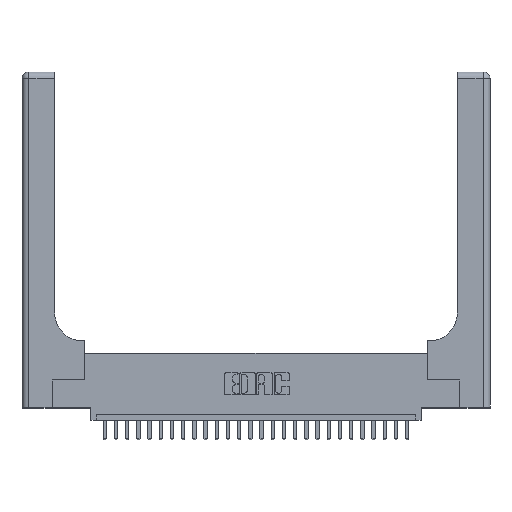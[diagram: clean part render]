
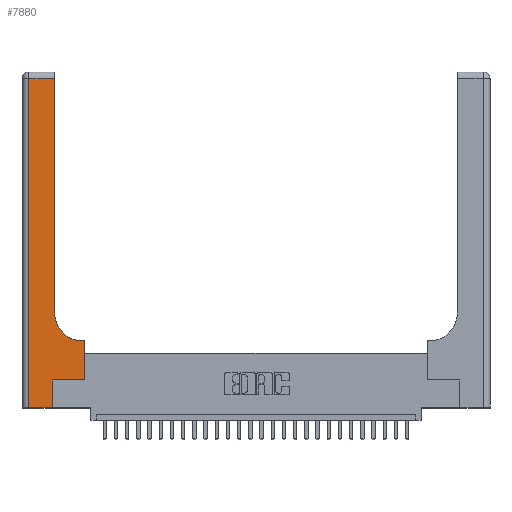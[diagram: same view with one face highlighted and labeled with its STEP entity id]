
A CAD part, top view. The second image highlights one B-rep face of the part: STEP entity #7880.
In plain terms, the highlighted planar face has unit normal (0, 0, 1).
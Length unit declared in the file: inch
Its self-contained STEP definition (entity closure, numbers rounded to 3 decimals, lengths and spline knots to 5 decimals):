
#289 = VECTOR ( 'NONE', #9527, 39.37008 ) ;
#341 = EDGE_CURVE ( 'NONE', #27066, #13692, #6060, .T. ) ;
#349 = ORIENTED_EDGE ( 'NONE', *, *, #12071, .T. ) ;
#788 = PLANE ( 'NONE',  #20138 ) ;
#1796 = VECTOR ( 'NONE', #8685, 39.37008 ) ;
#2355 = VERTEX_POINT ( 'NONE', #24753 ) ;
#2780 = VERTEX_POINT ( 'NONE', #15666 ) ;
#2901 = DIRECTION ( 'NONE',  ( 0., 0., -1. ) ) ;
#3776 = CARTESIAN_POINT ( 'NONE',  ( 0.06, 2.94, 0.37 ) ) ;
#3801 = CARTESIAN_POINT ( 'NONE',  ( 0., 0., 0.37 ) ) ;
#4126 = CARTESIAN_POINT ( 'NONE',  ( 0.06, 0., 0.37 ) ) ;
#4348 = VECTOR ( 'NONE', #10795, 39.37008 ) ;
#4604 = VERTEX_POINT ( 'NONE', #4126 ) ;
#4637 = VERTEX_POINT ( 'NONE', #7533 ) ;
#4756 = ORIENTED_EDGE ( 'NONE', *, *, #5649, .T. ) ;
#5040 = LINE ( 'NONE', #14088, #17760 ) ;
#5413 = FACE_OUTER_BOUND ( 'NONE', #22908, .T. ) ;
#5649 = EDGE_CURVE ( 'NONE', #4604, #4637, #25862, .T. ) ;
#5733 = LINE ( 'NONE', #9620, #289 ) ;
#6060 = LINE ( 'NONE', #28026, #4348 ) ;
#6322 = EDGE_CURVE ( 'NONE', #13692, #2355, #14817, .T. ) ;
#6333 = CARTESIAN_POINT ( 'NONE',  ( 0.5585, 0.25, 0.37 ) ) ;
#6763 = ORIENTED_EDGE ( 'NONE', *, *, #28104, .T. ) ;
#7533 = CARTESIAN_POINT ( 'NONE',  ( 0.269, 0., 0.37 ) ) ;
#7679 = VECTOR ( 'NONE', #20825, 39.37008 ) ;
#7880 = ADVANCED_FACE ( 'NONE', ( #5413 ), #788, .F. ) ;
#7980 = VERTEX_POINT ( 'NONE', #22956 ) ;
#8033 = CARTESIAN_POINT ( 'NONE',  ( 0.269, 0.25, 0.37 ) ) ;
#8475 = EDGE_CURVE ( 'NONE', #2355, #10216, #5040, .T. ) ;
#8685 = DIRECTION ( 'NONE',  ( 0., 1., 0. ) ) ;
#9446 = EDGE_CURVE ( 'NONE', #7980, #2780, #28351, .T. ) ;
#9454 = CARTESIAN_POINT ( 'NONE',  ( 0., 3., 0.37 ) ) ;
#9527 = DIRECTION ( 'NONE',  ( 0., -1., 0. ) ) ;
#9620 = CARTESIAN_POINT ( 'NONE',  ( 0.06, 3., 0.37 ) ) ;
#10079 = VECTOR ( 'NONE', #12360, 39.37008 ) ;
#10216 = VERTEX_POINT ( 'NONE', #26039 ) ;
#10705 = CIRCLE ( 'NONE', #15044, 0.25 ) ;
#10795 = DIRECTION ( 'NONE',  ( 1., 0., 0. ) ) ;
#12025 = CARTESIAN_POINT ( 'NONE',  ( 0.2915, 3., 0.37 ) ) ;
#12063 = LINE ( 'NONE', #13837, #25147 ) ;
#12071 = EDGE_CURVE ( 'NONE', #19812, #4604, #5733, .T. ) ;
#12283 = ORIENTED_EDGE ( 'NONE', *, *, #8475, .T. ) ;
#12360 = DIRECTION ( 'NONE',  ( 1., 0., 0. ) ) ;
#13520 = LINE ( 'NONE', #14239, #7679 ) ;
#13692 = VERTEX_POINT ( 'NONE', #14821 ) ;
#13837 = CARTESIAN_POINT ( 'NONE',  ( 0.269, 0., 0.37 ) ) ;
#13937 = DIRECTION ( 'NONE',  ( -1., 0., 0. ) ) ;
#14088 = CARTESIAN_POINT ( 'NONE',  ( 0.2915, 0.6, 0.37 ) ) ;
#14239 = CARTESIAN_POINT ( 'NONE',  ( 0., 2.94, 0.37 ) ) ;
#14691 = ORIENTED_EDGE ( 'NONE', *, *, #9446, .T. ) ;
#14753 = ORIENTED_EDGE ( 'NONE', *, *, #18419, .T. ) ;
#14817 = LINE ( 'NONE', #6333, #1796 ) ;
#14821 = CARTESIAN_POINT ( 'NONE',  ( 0.5585, 0.25, 0.37 ) ) ;
#15044 = AXIS2_PLACEMENT_3D ( 'NONE', #22582, #20565, #20386 ) ;
#15666 = CARTESIAN_POINT ( 'NONE',  ( 0.2915, 2.94, 0.37 ) ) ;
#15929 = DIRECTION ( 'NONE',  ( 0., 1., 0. ) ) ;
#16048 = ORIENTED_EDGE ( 'NONE', *, *, #27397, .T. ) ;
#17760 = VECTOR ( 'NONE', #24758, 39.37008 ) ;
#18419 = EDGE_CURVE ( 'NONE', #2780, #19812, #13520, .T. ) ;
#19049 = ORIENTED_EDGE ( 'NONE', *, *, #341, .T. ) ;
#19812 = VERTEX_POINT ( 'NONE', #3776 ) ;
#20138 = AXIS2_PLACEMENT_3D ( 'NONE', #9454, #2901, #13937 ) ;
#20386 = DIRECTION ( 'NONE',  ( 1., 0., 0. ) ) ;
#20565 = DIRECTION ( 'NONE',  ( 0., 0., -1. ) ) ;
#20825 = DIRECTION ( 'NONE',  ( -1., 0., 0. ) ) ;
#21129 = DIRECTION ( 'NONE',  ( 0., 1., 0. ) ) ;
#21890 = ORIENTED_EDGE ( 'NONE', *, *, #6322, .T. ) ;
#22523 = VECTOR ( 'NONE', #21129, 39.37008 ) ;
#22582 = CARTESIAN_POINT ( 'NONE',  ( 0.5415, 0.85, 0.37 ) ) ;
#22908 = EDGE_LOOP ( 'NONE', ( #14691, #14753, #349, #4756, #6763, #19049, #21890, #12283, #16048 ) ) ;
#22956 = CARTESIAN_POINT ( 'NONE',  ( 0.2915, 0.85, 0.37 ) ) ;
#24753 = CARTESIAN_POINT ( 'NONE',  ( 0.5585, 0.6, 0.37 ) ) ;
#24758 = DIRECTION ( 'NONE',  ( -1., 0., 0. ) ) ;
#25147 = VECTOR ( 'NONE', #15929, 39.37008 ) ;
#25862 = LINE ( 'NONE', #3801, #10079 ) ;
#26039 = CARTESIAN_POINT ( 'NONE',  ( 0.5415, 0.6, 0.37 ) ) ;
#27066 = VERTEX_POINT ( 'NONE', #8033 ) ;
#27397 = EDGE_CURVE ( 'NONE', #10216, #7980, #10705, .T. ) ;
#28026 = CARTESIAN_POINT ( 'NONE',  ( 0.269, 0.25, 0.37 ) ) ;
#28104 = EDGE_CURVE ( 'NONE', #4637, #27066, #12063, .T. ) ;
#28351 = LINE ( 'NONE', #12025, #22523 ) ;
